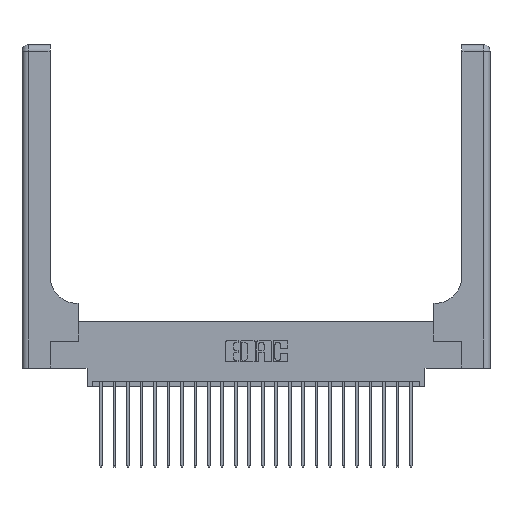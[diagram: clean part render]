
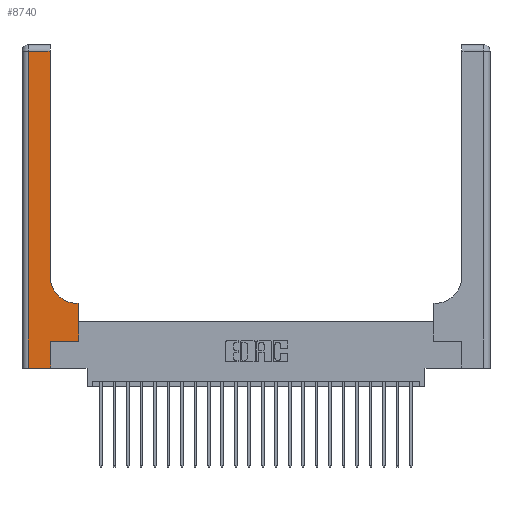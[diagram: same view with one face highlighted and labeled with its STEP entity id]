
A CAD part, top view. The second image highlights one B-rep face of the part: STEP entity #8740.
In plain terms, the highlighted planar face has unit normal (0, 0, 1).
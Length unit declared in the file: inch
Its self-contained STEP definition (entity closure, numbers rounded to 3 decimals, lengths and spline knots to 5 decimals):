
#252 = CARTESIAN_POINT ( 'NONE',  ( 0.528, 0.25, 0.37 ) ) ;
#585 = CARTESIAN_POINT ( 'NONE',  ( 0.265, 0.25, 0.37 ) ) ;
#916 = DIRECTION ( 'NONE',  ( 0., 0., -1. ) ) ;
#1348 = DIRECTION ( 'NONE',  ( -1., 0., 0. ) ) ;
#2084 = DIRECTION ( 'NONE',  ( 1., 0., 0. ) ) ;
#2356 = LINE ( 'NONE', #9619, #14000 ) ;
#2754 = VECTOR ( 'NONE', #23639, 39.37008 ) ;
#2921 = ORIENTED_EDGE ( 'NONE', *, *, #20424, .T. ) ;
#2945 = VERTEX_POINT ( 'NONE', #585 ) ;
#2967 = PLANE ( 'NONE',  #10490 ) ;
#3932 = VECTOR ( 'NONE', #18833, 39.37008 ) ;
#4039 = VERTEX_POINT ( 'NONE', #19132 ) ;
#4059 = DIRECTION ( 'NONE',  ( 0., -1., 0. ) ) ;
#5475 = AXIS2_PLACEMENT_3D ( 'NONE', #22114, #16309, #22235 ) ;
#6095 = EDGE_CURVE ( 'NONE', #13272, #13844, #22206, .T. ) ;
#6694 = EDGE_CURVE ( 'NONE', #2945, #4039, #16699, .T. ) ;
#6912 = EDGE_CURVE ( 'NONE', #6923, #13272, #9659, .T. ) ;
#6923 = VERTEX_POINT ( 'NONE', #13041 ) ;
#6987 = LINE ( 'NONE', #8805, #13696 ) ;
#7399 = VECTOR ( 'NONE', #2084, 39.37008 ) ;
#7454 = EDGE_LOOP ( 'NONE', ( #16797, #18516, #19100, #14828, #16021, #11896, #21982, #2921, #17500 ) ) ;
#7478 = VECTOR ( 'NONE', #19172, 39.37008 ) ;
#7611 = CARTESIAN_POINT ( 'NONE',  ( 0.26, 3., 0.37 ) ) ;
#7750 = EDGE_CURVE ( 'NONE', #4039, #12546, #15245, .T. ) ;
#7955 = CARTESIAN_POINT ( 'NONE',  ( 0.528, 0.6, 0.37 ) ) ;
#8740 = ADVANCED_FACE ( 'NONE', ( #10102 ), #2967, .F. ) ;
#8805 = CARTESIAN_POINT ( 'NONE',  ( 0., 0., 0.37 ) ) ;
#9033 = CARTESIAN_POINT ( 'NONE',  ( 0., 2.94, 0.37 ) ) ;
#9234 = EDGE_CURVE ( 'NONE', #11365, #6923, #15898, .T. ) ;
#9619 = CARTESIAN_POINT ( 'NONE',  ( 0.06, 3., 0.37 ) ) ;
#9659 = LINE ( 'NONE', #7611, #3932 ) ;
#10102 = FACE_OUTER_BOUND ( 'NONE', #7454, .T. ) ;
#10347 = CARTESIAN_POINT ( 'NONE',  ( 0., 3., 0.37 ) ) ;
#10490 = AXIS2_PLACEMENT_3D ( 'NONE', #10347, #916, #13852 ) ;
#11365 = VERTEX_POINT ( 'NONE', #17827 ) ;
#11727 = CARTESIAN_POINT ( 'NONE',  ( 0.06, 0., 0.37 ) ) ;
#11896 = ORIENTED_EDGE ( 'NONE', *, *, #6694, .T. ) ;
#12071 = VERTEX_POINT ( 'NONE', #11727 ) ;
#12246 = EDGE_CURVE ( 'NONE', #12071, #14766, #6987, .T. ) ;
#12546 = VERTEX_POINT ( 'NONE', #7955 ) ;
#12618 = CARTESIAN_POINT ( 'NONE',  ( 0.26, 2.94, 0.37 ) ) ;
#13041 = CARTESIAN_POINT ( 'NONE',  ( 0.26, 0.85, 0.37 ) ) ;
#13272 = VERTEX_POINT ( 'NONE', #12618 ) ;
#13696 = VECTOR ( 'NONE', #14361, 39.37008 ) ;
#13844 = VERTEX_POINT ( 'NONE', #19414 ) ;
#13852 = DIRECTION ( 'NONE',  ( -1., 0., 0. ) ) ;
#14000 = VECTOR ( 'NONE', #4059, 39.37008 ) ;
#14202 = EDGE_CURVE ( 'NONE', #13844, #12071, #2356, .T. ) ;
#14361 = DIRECTION ( 'NONE',  ( 1., 0., 0. ) ) ;
#14766 = VERTEX_POINT ( 'NONE', #20898 ) ;
#14828 = ORIENTED_EDGE ( 'NONE', *, *, #12246, .T. ) ;
#15245 = LINE ( 'NONE', #252, #21285 ) ;
#15588 = EDGE_CURVE ( 'NONE', #14766, #2945, #17478, .T. ) ;
#15898 = CIRCLE ( 'NONE', #5475, 0.25 ) ;
#16021 = ORIENTED_EDGE ( 'NONE', *, *, #15588, .T. ) ;
#16093 = LINE ( 'NONE', #20309, #16754 ) ;
#16309 = DIRECTION ( 'NONE',  ( 0., 0., -1. ) ) ;
#16699 = LINE ( 'NONE', #18760, #7399 ) ;
#16754 = VECTOR ( 'NONE', #1348, 39.37008 ) ;
#16797 = ORIENTED_EDGE ( 'NONE', *, *, #6912, .T. ) ;
#17478 = LINE ( 'NONE', #17720, #7478 ) ;
#17500 = ORIENTED_EDGE ( 'NONE', *, *, #9234, .T. ) ;
#17720 = CARTESIAN_POINT ( 'NONE',  ( 0.265, 0., 0.37 ) ) ;
#17827 = CARTESIAN_POINT ( 'NONE',  ( 0.51, 0.6, 0.37 ) ) ;
#18516 = ORIENTED_EDGE ( 'NONE', *, *, #6095, .T. ) ;
#18760 = CARTESIAN_POINT ( 'NONE',  ( 0.265, 0.25, 0.37 ) ) ;
#18833 = DIRECTION ( 'NONE',  ( 0., 1., 0. ) ) ;
#19100 = ORIENTED_EDGE ( 'NONE', *, *, #14202, .T. ) ;
#19132 = CARTESIAN_POINT ( 'NONE',  ( 0.528, 0.25, 0.37 ) ) ;
#19172 = DIRECTION ( 'NONE',  ( 0., 1., 0. ) ) ;
#19414 = CARTESIAN_POINT ( 'NONE',  ( 0.06, 2.94, 0.37 ) ) ;
#20309 = CARTESIAN_POINT ( 'NONE',  ( 0.26, 0.6, 0.37 ) ) ;
#20424 = EDGE_CURVE ( 'NONE', #12546, #11365, #16093, .T. ) ;
#20898 = CARTESIAN_POINT ( 'NONE',  ( 0.265, 0., 0.37 ) ) ;
#21285 = VECTOR ( 'NONE', #22495, 39.37008 ) ;
#21982 = ORIENTED_EDGE ( 'NONE', *, *, #7750, .T. ) ;
#22114 = CARTESIAN_POINT ( 'NONE',  ( 0.51, 0.85, 0.37 ) ) ;
#22206 = LINE ( 'NONE', #9033, #2754 ) ;
#22235 = DIRECTION ( 'NONE',  ( 1., 0., 0. ) ) ;
#22495 = DIRECTION ( 'NONE',  ( 0., 1., 0. ) ) ;
#23639 = DIRECTION ( 'NONE',  ( -1., 0., 0. ) ) ;
